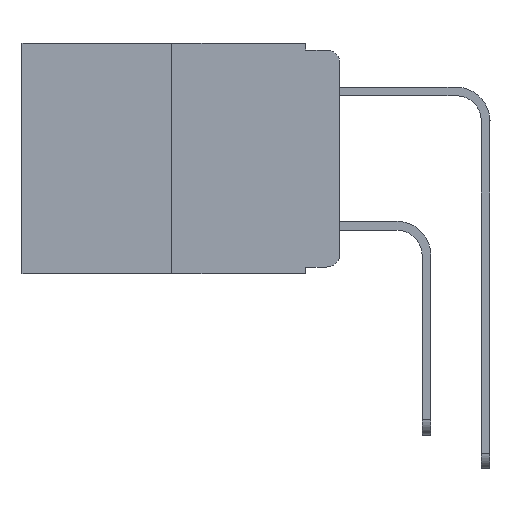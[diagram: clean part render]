
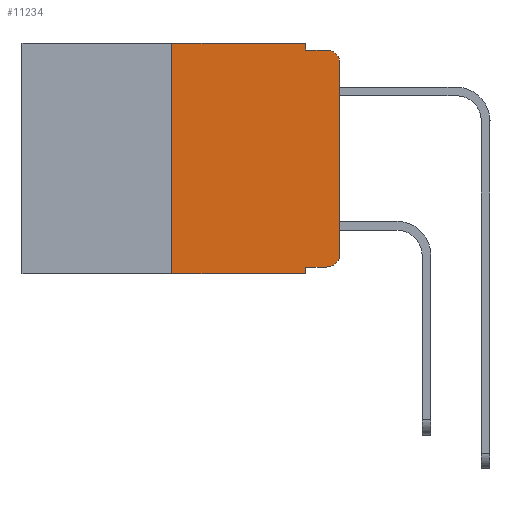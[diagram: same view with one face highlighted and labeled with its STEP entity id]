
A CAD part, left-side view. The second image highlights one B-rep face of the part: STEP entity #11234.
In plain terms, the highlighted planar face has unit normal (-1, 0, 0).
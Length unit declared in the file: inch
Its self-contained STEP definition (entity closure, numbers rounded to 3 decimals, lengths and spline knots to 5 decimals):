
#255 = DIRECTION ( 'NONE',  ( 0., 0., -1. ) ) ;
#490 = PLANE ( 'NONE',  #9441 ) ;
#566 = EDGE_CURVE ( 'NONE', #5840, #4465, #12107, .T. ) ;
#1186 = VERTEX_POINT ( 'NONE', #10592 ) ;
#1259 = CARTESIAN_POINT ( 'NONE',  ( 0., 0.25, 0. ) ) ;
#1592 = VERTEX_POINT ( 'NONE', #4102 ) ;
#1596 = LINE ( 'NONE', #5116, #7548 ) ;
#1754 = ORIENTED_EDGE ( 'NONE', *, *, #3557, .F. ) ;
#1777 = VERTEX_POINT ( 'NONE', #4335 ) ;
#2040 = VECTOR ( 'NONE', #7603, 39.37008 ) ;
#2300 = EDGE_LOOP ( 'NONE', ( #14002, #12338, #12645, #13671, #4453, #1754, #8362, #4095, #6622, #2511 ) ) ;
#2413 = LINE ( 'NONE', #4346, #2040 ) ;
#2463 = VERTEX_POINT ( 'NONE', #11994 ) ;
#2511 = ORIENTED_EDGE ( 'NONE', *, *, #566, .T. ) ;
#2578 = LINE ( 'NONE', #11982, #13897 ) ;
#2877 = CARTESIAN_POINT ( 'NONE',  ( 0., 0., 0. ) ) ;
#2880 = EDGE_CURVE ( 'NONE', #2463, #9837, #5755, .T. ) ;
#2934 = DIRECTION ( 'NONE',  ( 0., -1., 0. ) ) ;
#3557 = EDGE_CURVE ( 'NONE', #1592, #9778, #12084, .T. ) ;
#3894 = DIRECTION ( 'NONE',  ( 0., -1., 0. ) ) ;
#3948 = CARTESIAN_POINT ( 'NONE',  ( 0., 0.051, 0. ) ) ;
#4086 = CARTESIAN_POINT ( 'NONE',  ( 0., 0.473, 0. ) ) ;
#4095 = ORIENTED_EDGE ( 'NONE', *, *, #13424, .F. ) ;
#4102 = CARTESIAN_POINT ( 'NONE',  ( 0., 0.25, -0.343 ) ) ;
#4134 = DIRECTION ( 'NONE',  ( 0., 0., -1. ) ) ;
#4335 = CARTESIAN_POINT ( 'NONE',  ( 0., 0.051, -0.333 ) ) ;
#4346 = CARTESIAN_POINT ( 'NONE',  ( 0., 0.473, 0. ) ) ;
#4377 = EDGE_CURVE ( 'NONE', #9778, #2463, #2413, .T. ) ;
#4453 = ORIENTED_EDGE ( 'NONE', *, *, #4377, .F. ) ;
#4465 = VERTEX_POINT ( 'NONE', #11094 ) ;
#4560 = EDGE_CURVE ( 'NONE', #9146, #8022, #5891, .T. ) ;
#4709 = CARTESIAN_POINT ( 'NONE',  ( 0., 0.02, -0.03 ) ) ;
#5024 = EDGE_CURVE ( 'NONE', #9837, #8022, #2578, .T. ) ;
#5031 = FACE_OUTER_BOUND ( 'NONE', #2300, .T. ) ;
#5111 = DIRECTION ( 'NONE',  ( 0., 0., 1. ) ) ;
#5116 = CARTESIAN_POINT ( 'NONE',  ( 0., 0.051, -0.333 ) ) ;
#5674 = VECTOR ( 'NONE', #3894, 39.37008 ) ;
#5755 = LINE ( 'NONE', #3948, #11598 ) ;
#5807 = DIRECTION ( 'NONE',  ( 0., 0., -1. ) ) ;
#5840 = VERTEX_POINT ( 'NONE', #6518 ) ;
#5891 = CIRCLE ( 'NONE', #7825, 0.02 ) ;
#5896 = CARTESIAN_POINT ( 'NONE',  ( 0., 0., -0.03 ) ) ;
#6292 = EDGE_CURVE ( 'NONE', #4465, #9146, #7676, .T. ) ;
#6392 = AXIS2_PLACEMENT_3D ( 'NONE', #6601, #14248, #7700 ) ;
#6518 = CARTESIAN_POINT ( 'NONE',  ( 0., 0.02, -0.333 ) ) ;
#6601 = CARTESIAN_POINT ( 'NONE',  ( 0., 0.02, -0.313 ) ) ;
#6622 = ORIENTED_EDGE ( 'NONE', *, *, #11721, .T. ) ;
#6672 = LINE ( 'NONE', #9376, #5674 ) ;
#7131 = CARTESIAN_POINT ( 'NONE',  ( 0., 0.051, 0. ) ) ;
#7548 = VECTOR ( 'NONE', #2934, 39.37008 ) ;
#7603 = DIRECTION ( 'NONE',  ( 0., -1., 0. ) ) ;
#7676 = LINE ( 'NONE', #2877, #13169 ) ;
#7700 = DIRECTION ( 'NONE',  ( 0., 0., -1. ) ) ;
#7825 = AXIS2_PLACEMENT_3D ( 'NONE', #4709, #12367, #5807 ) ;
#8022 = VERTEX_POINT ( 'NONE', #11484 ) ;
#8362 = ORIENTED_EDGE ( 'NONE', *, *, #12760, .T. ) ;
#9146 = VERTEX_POINT ( 'NONE', #5896 ) ;
#9194 = VECTOR ( 'NONE', #10697, 39.37008 ) ;
#9376 = CARTESIAN_POINT ( 'NONE',  ( 0., 0.473, -0.343 ) ) ;
#9429 = DIRECTION ( 'NONE',  ( 0., 0., -1. ) ) ;
#9441 = AXIS2_PLACEMENT_3D ( 'NONE', #4086, #10703, #4134 ) ;
#9617 = CARTESIAN_POINT ( 'NONE',  ( 0., 0.25, 0. ) ) ;
#9778 = VERTEX_POINT ( 'NONE', #1259 ) ;
#9837 = VERTEX_POINT ( 'NONE', #12712 ) ;
#10592 = CARTESIAN_POINT ( 'NONE',  ( 0., 0.051, -0.343 ) ) ;
#10697 = DIRECTION ( 'NONE',  ( 0., 0., 1. ) ) ;
#10703 = DIRECTION ( 'NONE',  ( 1., 0., 0. ) ) ;
#11094 = CARTESIAN_POINT ( 'NONE',  ( 0., 0., -0.313 ) ) ;
#11234 = ADVANCED_FACE ( 'NONE', ( #5031 ), #490, .F. ) ;
#11484 = CARTESIAN_POINT ( 'NONE',  ( 0., 0.02, -0.01 ) ) ;
#11598 = VECTOR ( 'NONE', #9429, 39.37008 ) ;
#11677 = VECTOR ( 'NONE', #255, 39.37008 ) ;
#11721 = EDGE_CURVE ( 'NONE', #1777, #5840, #1596, .T. ) ;
#11982 = CARTESIAN_POINT ( 'NONE',  ( 0., 0.051, -0.01 ) ) ;
#11994 = CARTESIAN_POINT ( 'NONE',  ( 0., 0.051, 0. ) ) ;
#12084 = LINE ( 'NONE', #9617, #9194 ) ;
#12107 = CIRCLE ( 'NONE', #6392, 0.02 ) ;
#12338 = ORIENTED_EDGE ( 'NONE', *, *, #4560, .T. ) ;
#12367 = DIRECTION ( 'NONE',  ( -1., 0., 0. ) ) ;
#12645 = ORIENTED_EDGE ( 'NONE', *, *, #5024, .F. ) ;
#12712 = CARTESIAN_POINT ( 'NONE',  ( 0., 0.051, -0.01 ) ) ;
#12760 = EDGE_CURVE ( 'NONE', #1592, #1186, #6672, .T. ) ;
#13058 = DIRECTION ( 'NONE',  ( 0., -1., 0. ) ) ;
#13169 = VECTOR ( 'NONE', #5111, 39.37008 ) ;
#13424 = EDGE_CURVE ( 'NONE', #1777, #1186, #14180, .T. ) ;
#13671 = ORIENTED_EDGE ( 'NONE', *, *, #2880, .F. ) ;
#13897 = VECTOR ( 'NONE', #13058, 39.37008 ) ;
#14002 = ORIENTED_EDGE ( 'NONE', *, *, #6292, .T. ) ;
#14180 = LINE ( 'NONE', #7131, #11677 ) ;
#14248 = DIRECTION ( 'NONE',  ( -1., 0., 0. ) ) ;
